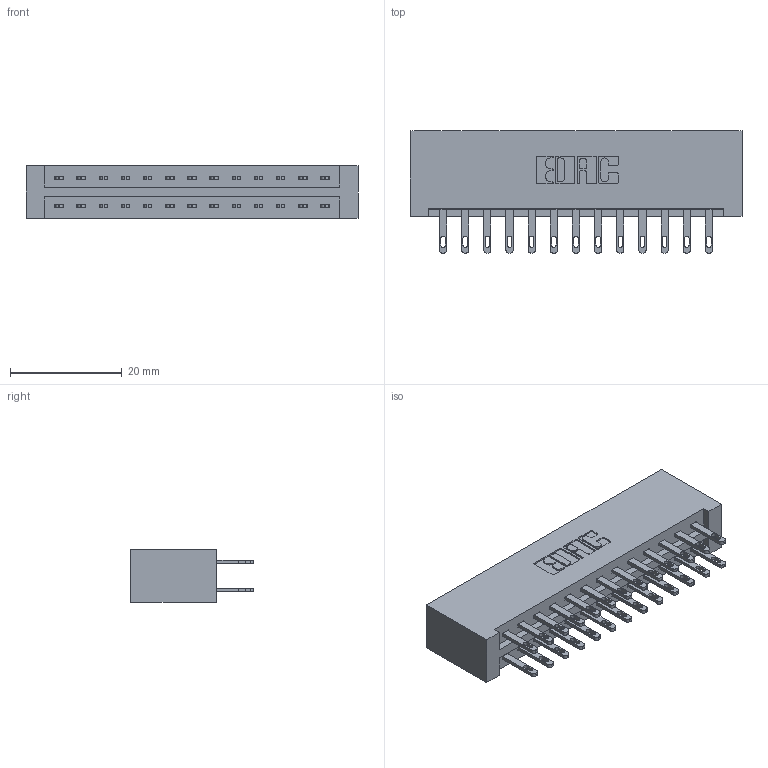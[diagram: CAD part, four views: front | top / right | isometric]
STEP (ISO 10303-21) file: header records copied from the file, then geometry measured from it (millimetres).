
FILE_DESCRIPTION (( 'STEP AP203' ), '1' );
FILE_NAME ('337-026-500-201.STEP', '2019-10-08T15:51:49', ( '' ), ( '' ), 'SwSTEP 2.0', 'SolidWorks 2016', '' );
FILE_SCHEMA (( 'CONFIG_CONTROL_DESIGN' ));
Length unit declared in the file: inch
Products named in the file (3): 337 Part_No Mounting Lugs; 345-292-001_345-293-100; 337-026-500-201
Assembly tree (27 placements, depth 2):
  337-026-500-201
    337 Part_No Mounting Lugs
    345-292-001_345-293-100  x26
Bounding box: 59.39 x 21.85 x 9.4 mm (x, y, z)
Volume: 6712.7 mm3; surface area: 7651.6 mm2
Topology: 27 solids, 27 shells, 1406 faces, 4265 edges, 2842 vertices
Faces by surface type: plane 898, cylinder 508
Entity records: 13483 total; most frequent: CARTESIAN_POINT 2294, ORIENTED_EDGE 2230, DIRECTION 1999, EDGE_CURVE 1115, LINE 991, VECTOR 991, VERTEX_POINT 742, AXIS2_PLACEMENT_3D 504
